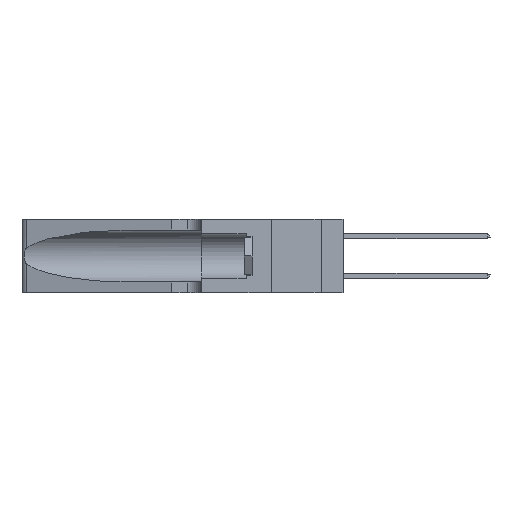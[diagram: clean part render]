
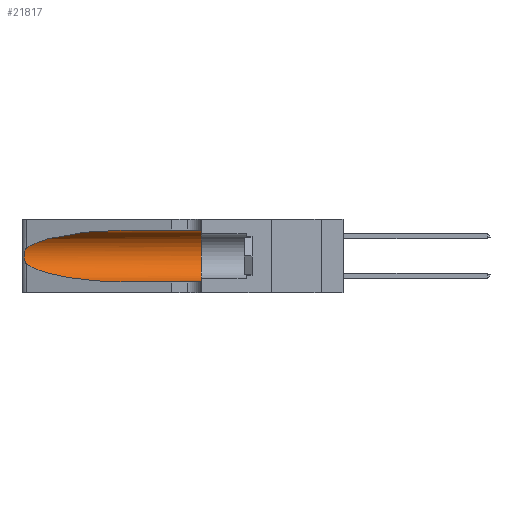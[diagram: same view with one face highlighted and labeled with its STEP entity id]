
A CAD part, left-side view. The second image highlights one B-rep face of the part: STEP entity #21817.
In plain terms, the highlighted cylindrical face has radius 3.308 mm (diameter 6.617 mm), a partial arc.
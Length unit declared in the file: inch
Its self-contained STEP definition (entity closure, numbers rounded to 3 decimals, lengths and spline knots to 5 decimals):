
#203 = VERTEX_POINT ( 'NONE', #7386 ) ;
#379 = CARTESIAN_POINT ( 'NONE',  ( 0.25487, 1.22718, 0.22369 ) ) ;
#1340 = FACE_OUTER_BOUND ( 'NONE', #35881, .T. ) ;
#1456 = CARTESIAN_POINT ( 'NONE',  ( 0.25639, 1.23184, 0.21858 ) ) ;
#1908 = DIRECTION ( 'NONE',  ( 0., 0., -1. ) ) ;
#2195 =( BOUNDED_CURVE ( )  B_SPLINE_CURVE ( 3, ( #6950, #27628, #9934, #30622 ),
 .UNSPECIFIED., .F., .F. ) 
 B_SPLINE_CURVE_WITH_KNOTS ( ( 4, 4 ),
 ( 3.44316, 4.71239 ),
 .UNSPECIFIED. ) 
 CURVE ( )  GEOMETRIC_REPRESENTATION_ITEM ( )  RATIONAL_B_SPLINE_CURVE ( ( 1., 0.87, 0.87, 1. ) ) 
 REPRESENTATION_ITEM ( '' )  );
#2564 = EDGE_CURVE ( 'NONE', #203, #32747, #2195, .T. ) ;
#3717 = CARTESIAN_POINT ( 'NONE',  ( 0.1305, 0.35, 0.185 ) ) ;
#4439 = CARTESIAN_POINT ( 'NONE',  ( 0.25854, 1.2359, 0.20912 ) ) ;
#6442 = CARTESIAN_POINT ( 'NONE',  ( 0.1305, 0.35, 0.05475 ) ) ;
#6685 = DIRECTION ( 'NONE',  ( 0., 0., 1. ) ) ;
#6950 = CARTESIAN_POINT ( 'NONE',  ( 0.25487, 1.22718, 0.14631 ) ) ;
#7345 = CYLINDRICAL_SURFACE ( 'NONE', #9735, 0.13025 ) ;
#7386 = CARTESIAN_POINT ( 'NONE',  ( 0.25487, 1.22718, 0.14631 ) ) ;
#7400 = CARTESIAN_POINT ( 'NONE',  ( 0.26075, 1.23896, 0.19203 ) ) ;
#8044 = ORIENTED_EDGE ( 'NONE', *, *, #31451, .F. ) ;
#8146 = VERTEX_POINT ( 'NONE', #16351 ) ;
#9551 = CARTESIAN_POINT ( 'NONE',  ( 0.1305, 0.72297, 0.31525 ) ) ;
#9735 = AXIS2_PLACEMENT_3D ( 'NONE', #37345, #31515, #1908 ) ;
#9934 = CARTESIAN_POINT ( 'NONE',  ( 0.18966, 0.96281, 0.05475 ) ) ;
#10393 = CARTESIAN_POINT ( 'NONE',  ( 0.26017, 1.23833, 0.17102 ) ) ;
#11549 = CARTESIAN_POINT ( 'NONE',  ( 0.1305, 0.35, 0.31525 ) ) ;
#12353 = B_SPLINE_CURVE_WITH_KNOTS ( 'NONE', 3,
 ( #16163, #36896, #1456, #22113, #4439, #25120, #7400, #28081, #10393, #31081, #13324, #34052, #16292, #37023 ),
 .UNSPECIFIED., .F., .F.,
 ( 4, 2, 2, 2, 2, 2, 4 ),
 ( 0., 0.00027, 0.00053, 0.00107, 0.0016, 0.00187, 0.00214 ),
 .UNSPECIFIED. ) ;
#13324 = CARTESIAN_POINT ( 'NONE',  ( 0.25789, 1.23486, 0.15765 ) ) ;
#15094 = CARTESIAN_POINT ( 'NONE',  ( 0.18966, 0.96281, 0.31525 ) ) ;
#16163 = CARTESIAN_POINT ( 'NONE',  ( 0.25487, 1.22718, 0.22369 ) ) ;
#16292 = CARTESIAN_POINT ( 'NONE',  ( 0.25555, 1.22993, 0.14849 ) ) ;
#16351 = CARTESIAN_POINT ( 'NONE',  ( 0.25487, 1.22718, 0.22369 ) ) ;
#16388 =( BOUNDED_CURVE ( )  B_SPLINE_CURVE ( 3, ( #23912, #15094, #18097, #379 ),
 .UNSPECIFIED., .F., .F. ) 
 B_SPLINE_CURVE_WITH_KNOTS ( ( 4, 4 ),
 ( 1.5708, 2.84003 ),
 .UNSPECIFIED. ) 
 CURVE ( )  GEOMETRIC_REPRESENTATION_ITEM ( )  RATIONAL_B_SPLINE_CURVE ( ( 1., 0.87, 0.87, 1. ) ) 
 REPRESENTATION_ITEM ( '' )  );
#17885 = EDGE_CURVE ( 'NONE', #31441, #8146, #16388, .T. ) ;
#18063 = VECTOR ( 'NONE', #27395, 39.37008 ) ;
#18097 = CARTESIAN_POINT ( 'NONE',  ( 0.2373, 1.15595, 0.28018 ) ) ;
#19754 = DIRECTION ( 'NONE',  ( 0., -1., 0. ) ) ;
#21424 = CARTESIAN_POINT ( 'NONE',  ( 0.1305, 1.61858, 0.05475 ) ) ;
#21817 = ADVANCED_FACE ( 'NONE', ( #1340 ), #7345, .F. ) ;
#22105 = ORIENTED_EDGE ( 'NONE', *, *, #33484, .T. ) ;
#22113 = CARTESIAN_POINT ( 'NONE',  ( 0.25787, 1.23484, 0.2124 ) ) ;
#23809 = LINE ( 'NONE', #37402, #32627 ) ;
#23912 = CARTESIAN_POINT ( 'NONE',  ( 0.1305, 0.72297, 0.31525 ) ) ;
#24054 = EDGE_CURVE ( 'NONE', #31441, #24900, #23809, .T. ) ;
#24356 = VERTEX_POINT ( 'NONE', #6442 ) ;
#24380 = DIRECTION ( 'NONE',  ( 0., 1., 0. ) ) ;
#24900 = VERTEX_POINT ( 'NONE', #11549 ) ;
#25120 = CARTESIAN_POINT ( 'NONE',  ( 0.26018, 1.23835, 0.19895 ) ) ;
#27395 = DIRECTION ( 'NONE',  ( 0., -1., 0. ) ) ;
#27628 = CARTESIAN_POINT ( 'NONE',  ( 0.2373, 1.15595, 0.08982 ) ) ;
#28081 = CARTESIAN_POINT ( 'NONE',  ( 0.26075, 1.23896, 0.178 ) ) ;
#29462 = ORIENTED_EDGE ( 'NONE', *, *, #24054, .F. ) ;
#30622 = CARTESIAN_POINT ( 'NONE',  ( 0.1305, 0.72297, 0.05475 ) ) ;
#31081 = CARTESIAN_POINT ( 'NONE',  ( 0.25856, 1.23593, 0.16098 ) ) ;
#31441 = VERTEX_POINT ( 'NONE', #9551 ) ;
#31451 = EDGE_CURVE ( 'NONE', #24900, #24356, #35234, .T. ) ;
#31515 = DIRECTION ( 'NONE',  ( 0., -1., 0. ) ) ;
#32627 = VECTOR ( 'NONE', #19754, 39.37008 ) ;
#32747 = VERTEX_POINT ( 'NONE', #33714 ) ;
#33484 = EDGE_CURVE ( 'NONE', #8146, #203, #12353, .T. ) ;
#33714 = CARTESIAN_POINT ( 'NONE',  ( 0.1305, 0.72297, 0.05475 ) ) ;
#34001 = EDGE_CURVE ( 'NONE', #32747, #24356, #35661, .T. ) ;
#34052 = CARTESIAN_POINT ( 'NONE',  ( 0.25639, 1.23186, 0.15144 ) ) ;
#35234 = CIRCLE ( 'NONE', #37445, 0.13025 ) ;
#35661 = LINE ( 'NONE', #21424, #18063 ) ;
#35881 = EDGE_LOOP ( 'NONE', ( #37414, #22105, #37341, #38195, #8044, #29462 ) ) ;
#36896 = CARTESIAN_POINT ( 'NONE',  ( 0.25555, 1.22994, 0.2215 ) ) ;
#37023 = CARTESIAN_POINT ( 'NONE',  ( 0.25487, 1.22718, 0.14631 ) ) ;
#37341 = ORIENTED_EDGE ( 'NONE', *, *, #2564, .T. ) ;
#37345 = CARTESIAN_POINT ( 'NONE',  ( 0.1305, 1.61858, 0.185 ) ) ;
#37402 = CARTESIAN_POINT ( 'NONE',  ( 0.1305, 1.61858, 0.31525 ) ) ;
#37414 = ORIENTED_EDGE ( 'NONE', *, *, #17885, .T. ) ;
#37445 = AXIS2_PLACEMENT_3D ( 'NONE', #3717, #24380, #6685 ) ;
#38195 = ORIENTED_EDGE ( 'NONE', *, *, #34001, .T. ) ;
